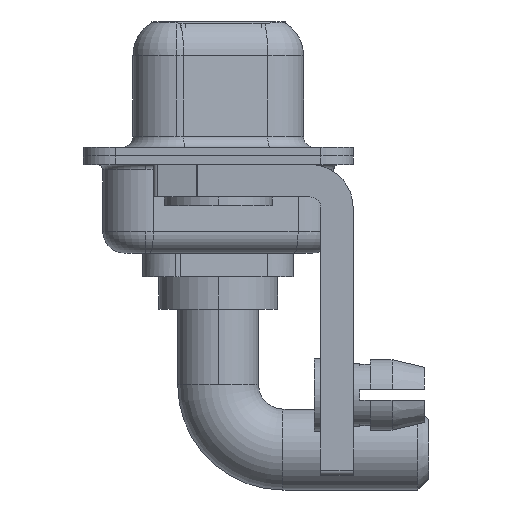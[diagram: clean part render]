
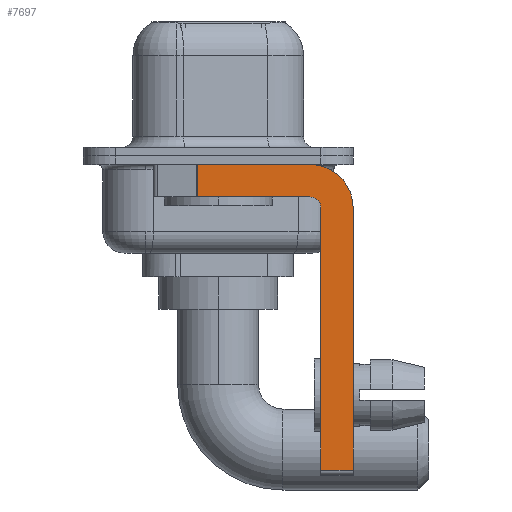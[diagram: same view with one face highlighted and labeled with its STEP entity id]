
A CAD part, left-side view. The second image highlights one B-rep face of the part: STEP entity #7697.
In plain terms, the highlighted planar face has unit normal (-1, 0, 0).
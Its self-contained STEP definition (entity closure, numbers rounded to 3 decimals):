
#15 = VERTEX_POINT ( 'NONE', #3214 ) ;
#214 = VECTOR ( 'NONE', #3395, 1000. ) ;
#260 = VERTEX_POINT ( 'NONE', #1556 ) ;
#435 = CARTESIAN_POINT ( 'NONE',  ( -2.9, -4.25, -14.55 ) ) ;
#467 = CARTESIAN_POINT ( 'NONE',  ( -2.9, -4.25, -2.4 ) ) ;
#519 = EDGE_LOOP ( 'NONE', ( #6064, #3186, #3932, #15186, #8244, #8778, #11964, #3739 ) ) ;
#644 = EDGE_CURVE ( 'NONE', #4220, #15, #2399, .T. ) ;
#1554 = LINE ( 'NONE', #435, #9470 ) ;
#1556 = CARTESIAN_POINT ( 'NONE',  ( -2.9, -4.75, -14.55 ) ) ;
#1952 = CARTESIAN_POINT ( 'NONE',  ( -2.9, -4.25, -2.4 ) ) ;
#2399 = LINE ( 'NONE', #14761, #2808 ) ;
#2618 = EDGE_CURVE ( 'NONE', #260, #5286, #9413, .T. ) ;
#2808 = VECTOR ( 'NONE', #10870, 1000. ) ;
#3161 = EDGE_CURVE ( 'NONE', #5286, #4220, #11785, .T. ) ;
#3186 = ORIENTED_EDGE ( 'NONE', *, *, #14768, .T. ) ;
#3214 = CARTESIAN_POINT ( 'NONE',  ( -2.9, 0.978, -1.9 ) ) ;
#3395 = DIRECTION ( 'NONE',  ( 0., 0., -1. ) ) ;
#3739 = ORIENTED_EDGE ( 'NONE', *, *, #11502, .F. ) ;
#3773 = CARTESIAN_POINT ( 'NONE',  ( -2.9, -4.25, -2.4 ) ) ;
#3932 = ORIENTED_EDGE ( 'NONE', *, *, #644, .F. ) ;
#4074 = CIRCLE ( 'NONE', #10635, 2. ) ;
#4183 = EDGE_CURVE ( 'NONE', #260, #4416, #1554, .T. ) ;
#4220 = VERTEX_POINT ( 'NONE', #8910 ) ;
#4242 = VECTOR ( 'NONE', #15675, 1000. ) ;
#4416 = VERTEX_POINT ( 'NONE', #8253 ) ;
#4590 = LINE ( 'NONE', #14255, #214 ) ;
#5217 = AXIS2_PLACEMENT_3D ( 'NONE', #3773, #9861, #7646 ) ;
#5272 = DIRECTION ( 'NONE',  ( 0., -1., 0. ) ) ;
#5286 = VERTEX_POINT ( 'NONE', #8305 ) ;
#5492 = VECTOR ( 'NONE', #15641, 1000. ) ;
#5880 = EDGE_CURVE ( 'NONE', #6804, #12936, #8132, .T. ) ;
#5946 = CARTESIAN_POINT ( 'NONE',  ( -2.9, -6.25, -2.4 ) ) ;
#6064 = ORIENTED_EDGE ( 'NONE', *, *, #5880, .F. ) ;
#6767 = DIRECTION ( 'NONE',  ( 1., 0., 0. ) ) ;
#6804 = VERTEX_POINT ( 'NONE', #12855 ) ;
#7307 = AXIS2_PLACEMENT_3D ( 'NONE', #467, #7968, #7662 ) ;
#7646 = DIRECTION ( 'NONE',  ( 0., 0., 1. ) ) ;
#7662 = DIRECTION ( 'NONE',  ( 0., 0., -1. ) ) ;
#7697 = ADVANCED_FACE ( 'NONE', ( #14884 ), #8857, .F. ) ;
#7968 = DIRECTION ( 'NONE',  ( 1., 0., 0. ) ) ;
#8132 = LINE ( 'NONE', #10876, #5492 ) ;
#8244 = ORIENTED_EDGE ( 'NONE', *, *, #2618, .F. ) ;
#8253 = CARTESIAN_POINT ( 'NONE',  ( -2.9, -6.25, -14.55 ) ) ;
#8305 = CARTESIAN_POINT ( 'NONE',  ( -2.9, -4.75, -2.4 ) ) ;
#8757 = LINE ( 'NONE', #13605, #4242 ) ;
#8778 = ORIENTED_EDGE ( 'NONE', *, *, #4183, .T. ) ;
#8857 = PLANE ( 'NONE',  #7307 ) ;
#8910 = CARTESIAN_POINT ( 'NONE',  ( -2.9, -4.25, -1.9 ) ) ;
#8927 = EDGE_CURVE ( 'NONE', #12726, #4416, #4590, .T. ) ;
#9340 = DIRECTION ( 'NONE',  ( 0., 0., 1. ) ) ;
#9413 = LINE ( 'NONE', #15297, #15539 ) ;
#9470 = VECTOR ( 'NONE', #5272, 1000. ) ;
#9861 = DIRECTION ( 'NONE',  ( -1., 0., 0. ) ) ;
#10420 = DIRECTION ( 'NONE',  ( 0., 0., -1. ) ) ;
#10635 = AXIS2_PLACEMENT_3D ( 'NONE', #1952, #6767, #10420 ) ;
#10870 = DIRECTION ( 'NONE',  ( 0., 1., 0. ) ) ;
#10876 = CARTESIAN_POINT ( 'NONE',  ( -2.9, 3., -0.4 ) ) ;
#11502 = EDGE_CURVE ( 'NONE', #12936, #12726, #4074, .T. ) ;
#11785 = CIRCLE ( 'NONE', #5217, 0.5 ) ;
#11964 = ORIENTED_EDGE ( 'NONE', *, *, #8927, .F. ) ;
#12726 = VERTEX_POINT ( 'NONE', #5946 ) ;
#12855 = CARTESIAN_POINT ( 'NONE',  ( -2.9, 0.978, -0.4 ) ) ;
#12936 = VERTEX_POINT ( 'NONE', #14987 ) ;
#13605 = CARTESIAN_POINT ( 'NONE',  ( -2.9, 0.978, -1.9 ) ) ;
#14255 = CARTESIAN_POINT ( 'NONE',  ( -2.9, -6.25, -2.4 ) ) ;
#14761 = CARTESIAN_POINT ( 'NONE',  ( -2.9, -4.25, -1.9 ) ) ;
#14768 = EDGE_CURVE ( 'NONE', #6804, #15, #8757, .T. ) ;
#14884 = FACE_OUTER_BOUND ( 'NONE', #519, .T. ) ;
#14987 = CARTESIAN_POINT ( 'NONE',  ( -2.9, -4.25, -0.4 ) ) ;
#15186 = ORIENTED_EDGE ( 'NONE', *, *, #3161, .F. ) ;
#15297 = CARTESIAN_POINT ( 'NONE',  ( -2.9, -4.75, -14.8 ) ) ;
#15539 = VECTOR ( 'NONE', #9340, 1000. ) ;
#15641 = DIRECTION ( 'NONE',  ( 0., -1., 0. ) ) ;
#15675 = DIRECTION ( 'NONE',  ( 0., 0., -1. ) ) ;
